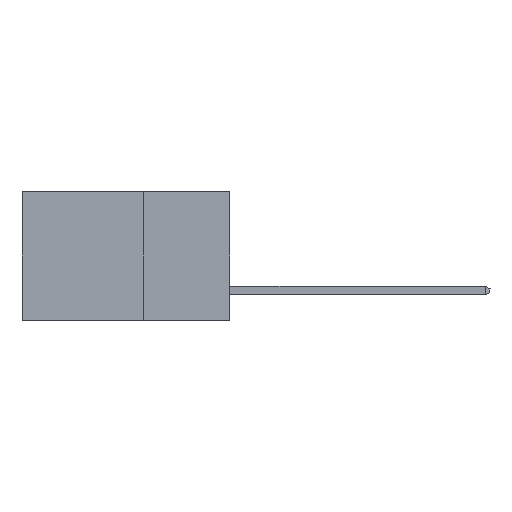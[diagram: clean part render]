
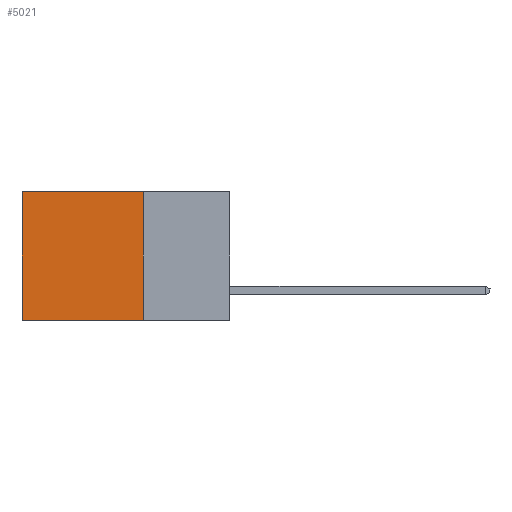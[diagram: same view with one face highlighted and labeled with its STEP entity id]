
A CAD part, left-side view. The second image highlights one B-rep face of the part: STEP entity #5021.
In plain terms, the highlighted planar face has unit normal (-1, 0, 0).
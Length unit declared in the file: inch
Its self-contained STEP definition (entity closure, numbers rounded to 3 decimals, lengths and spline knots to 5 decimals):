
#69 = ORIENTED_EDGE ( 'NONE', *, *, #8915, .F. ) ;
#91 = ORIENTED_EDGE ( 'NONE', *, *, #5170, .T. ) ;
#206 = ORIENTED_EDGE ( 'NONE', *, *, #10327, .T. ) ;
#881 = VECTOR ( 'NONE', #2412, 39.37008 ) ;
#897 = CARTESIAN_POINT ( 'NONE',  ( 0.298, 0.6, -0.37 ) ) ;
#1195 = VERTEX_POINT ( 'NONE', #897 ) ;
#2157 = CARTESIAN_POINT ( 'NONE',  ( 0.298, 0.6, 0. ) ) ;
#2412 = DIRECTION ( 'NONE',  ( 0., 0., -1. ) ) ;
#2482 = AXIS2_PLACEMENT_3D ( 'NONE', #9547, #4012, #10477 ) ;
#2986 = ORIENTED_EDGE ( 'NONE', *, *, #9919, .F. ) ;
#3084 = PLANE ( 'NONE',  #2482 ) ;
#3223 = VERTEX_POINT ( 'NONE', #10804 ) ;
#3504 = LINE ( 'NONE', #9558, #8003 ) ;
#3867 = DIRECTION ( 'NONE',  ( 0., 0., -1. ) ) ;
#3930 = LINE ( 'NONE', #10757, #7997 ) ;
#4012 = DIRECTION ( 'NONE',  ( 1., 0., 0. ) ) ;
#4626 = FACE_OUTER_BOUND ( 'NONE', #5824, .T. ) ;
#5021 = ADVANCED_FACE ( 'NONE', ( #4626 ), #3084, .F. ) ;
#5170 = EDGE_CURVE ( 'NONE', #3223, #8874, #10396, .T. ) ;
#5824 = EDGE_LOOP ( 'NONE', ( #206, #2986, #69, #91 ) ) ;
#6088 = LINE ( 'NONE', #8009, #881 ) ;
#7360 = CARTESIAN_POINT ( 'NONE',  ( 0.298, 0.25, -0.37 ) ) ;
#7614 = VERTEX_POINT ( 'NONE', #7360 ) ;
#7865 = CARTESIAN_POINT ( 'NONE',  ( 0.298, 0.25, 0. ) ) ;
#7997 = VECTOR ( 'NONE', #9873, 39.37008 ) ;
#8003 = VECTOR ( 'NONE', #3867, 39.37008 ) ;
#8009 = CARTESIAN_POINT ( 'NONE',  ( 0.298, 0.6, 0. ) ) ;
#8874 = VERTEX_POINT ( 'NONE', #2157 ) ;
#8915 = EDGE_CURVE ( 'NONE', #3223, #7614, #3504, .T. ) ;
#9547 = CARTESIAN_POINT ( 'NONE',  ( 0.298, 0.25, 0. ) ) ;
#9558 = CARTESIAN_POINT ( 'NONE',  ( 0.298, 0.25, 0. ) ) ;
#9873 = DIRECTION ( 'NONE',  ( 0., 1., 0. ) ) ;
#9919 = EDGE_CURVE ( 'NONE', #7614, #1195, #3930, .T. ) ;
#10116 = VECTOR ( 'NONE', #10683, 39.37008 ) ;
#10327 = EDGE_CURVE ( 'NONE', #8874, #1195, #6088, .T. ) ;
#10396 = LINE ( 'NONE', #7865, #10116 ) ;
#10477 = DIRECTION ( 'NONE',  ( 0., 0., -1. ) ) ;
#10683 = DIRECTION ( 'NONE',  ( 0., 1., 0. ) ) ;
#10757 = CARTESIAN_POINT ( 'NONE',  ( 0.298, 0.25, -0.37 ) ) ;
#10804 = CARTESIAN_POINT ( 'NONE',  ( 0.298, 0.25, 0. ) ) ;
